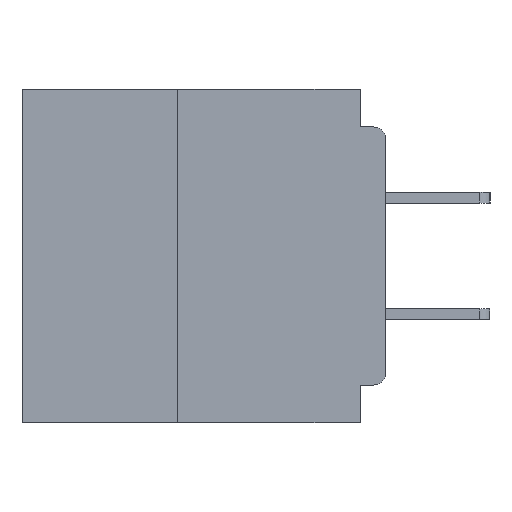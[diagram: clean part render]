
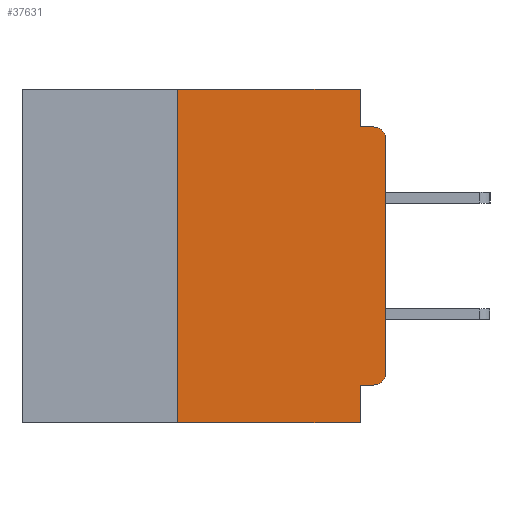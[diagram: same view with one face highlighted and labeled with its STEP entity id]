
A CAD part, left-side view. The second image highlights one B-rep face of the part: STEP entity #37631.
In plain terms, the highlighted planar face has unit normal (-1, 0, 0).
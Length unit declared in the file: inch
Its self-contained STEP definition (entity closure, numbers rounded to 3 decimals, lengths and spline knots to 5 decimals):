
#302 = DIRECTION ( 'NONE',  ( 0., 0., 1. ) ) ;
#959 = DIRECTION ( 'NONE',  ( 0., 0., -1. ) ) ;
#1338 = CARTESIAN_POINT ( 'NONE',  ( 0., 0.015, -0.045 ) ) ;
#1411 = ORIENTED_EDGE ( 'NONE', *, *, #16691, .T. ) ;
#1636 = VERTEX_POINT ( 'NONE', #13300 ) ;
#2552 = CARTESIAN_POINT ( 'NONE',  ( 0., 0.031, -0.4 ) ) ;
#2726 = VERTEX_POINT ( 'NONE', #1338 ) ;
#2742 = LINE ( 'NONE', #43406, #20763 ) ;
#3645 = VERTEX_POINT ( 'NONE', #13835 ) ;
#4211 = DIRECTION ( 'NONE',  ( 0., 0., -1. ) ) ;
#4636 = CARTESIAN_POINT ( 'NONE',  ( 0., 0.25, -0.4 ) ) ;
#4673 = CARTESIAN_POINT ( 'NONE',  ( 0., 0.031, 0. ) ) ;
#4762 = EDGE_CURVE ( 'NONE', #6671, #3645, #5255, .T. ) ;
#5042 = VECTOR ( 'NONE', #33403, 39.37008 ) ;
#5255 = LINE ( 'NONE', #2552, #23279 ) ;
#6236 = ORIENTED_EDGE ( 'NONE', *, *, #14813, .F. ) ;
#6671 = VERTEX_POINT ( 'NONE', #9232 ) ;
#7798 = ORIENTED_EDGE ( 'NONE', *, *, #25783, .T. ) ;
#8801 = DIRECTION ( 'NONE',  ( 0., 1., 0. ) ) ;
#9017 = VECTOR ( 'NONE', #30802, 39.37008 ) ;
#9232 = CARTESIAN_POINT ( 'NONE',  ( 0., 0.031, -0.355 ) ) ;
#9475 = AXIS2_PLACEMENT_3D ( 'NONE', #44064, #22482, #959 ) ;
#9657 = AXIS2_PLACEMENT_3D ( 'NONE', #11304, #25744, #4211 ) ;
#10311 = LINE ( 'NONE', #16710, #27148 ) ;
#11252 = LINE ( 'NONE', #22728, #5042 ) ;
#11304 = CARTESIAN_POINT ( 'NONE',  ( 0., 0.437, 0. ) ) ;
#11987 = LINE ( 'NONE', #4636, #20403 ) ;
#13208 = CARTESIAN_POINT ( 'NONE',  ( 0., 0.25, 0. ) ) ;
#13300 = CARTESIAN_POINT ( 'NONE',  ( 0., 0., -0.06 ) ) ;
#13835 = CARTESIAN_POINT ( 'NONE',  ( 0., 0.031, -0.4 ) ) ;
#14813 = EDGE_CURVE ( 'NONE', #42916, #33539, #35148, .T. ) ;
#16017 = VECTOR ( 'NONE', #8801, 39.37008 ) ;
#16586 = VERTEX_POINT ( 'NONE', #29084 ) ;
#16691 = EDGE_CURVE ( 'NONE', #1636, #2726, #40335, .T. ) ;
#16710 = CARTESIAN_POINT ( 'NONE',  ( 0., 0.437, 0. ) ) ;
#18535 = PLANE ( 'NONE',  #9657 ) ;
#18808 = VERTEX_POINT ( 'NONE', #13208 ) ;
#19559 = EDGE_CURVE ( 'NONE', #18808, #42916, #10311, .T. ) ;
#19618 = ORIENTED_EDGE ( 'NONE', *, *, #23415, .F. ) ;
#19667 = CARTESIAN_POINT ( 'NONE',  ( 0., 0.015, -0.355 ) ) ;
#20085 = CARTESIAN_POINT ( 'NONE',  ( 0., 0.015, -0.34 ) ) ;
#20403 = VECTOR ( 'NONE', #33405, 39.37008 ) ;
#20763 = VECTOR ( 'NONE', #302, 39.37008 ) ;
#20807 = EDGE_LOOP ( 'NONE', ( #30777, #1411, #39521, #6236, #39574, #31554, #7798, #27326, #19618, #28638 ) ) ;
#22482 = DIRECTION ( 'NONE',  ( -1., 0., 0. ) ) ;
#22728 = CARTESIAN_POINT ( 'NONE',  ( 0., 0., -0.045 ) ) ;
#23279 = VECTOR ( 'NONE', #24097, 39.37008 ) ;
#23415 = EDGE_CURVE ( 'NONE', #39044, #6671, #35107, .T. ) ;
#23688 = DIRECTION ( 'NONE',  ( 0., 0., -1. ) ) ;
#24097 = DIRECTION ( 'NONE',  ( 0., 0., -1. ) ) ;
#25744 = DIRECTION ( 'NONE',  ( 1., 0., 0. ) ) ;
#25758 = AXIS2_PLACEMENT_3D ( 'NONE', #20085, #45265, #23688 ) ;
#25783 = EDGE_CURVE ( 'NONE', #39995, #3645, #36567, .T. ) ;
#26922 = FACE_OUTER_BOUND ( 'NONE', #20807, .T. ) ;
#27148 = VECTOR ( 'NONE', #41887, 39.37008 ) ;
#27326 = ORIENTED_EDGE ( 'NONE', *, *, #4762, .F. ) ;
#28638 = ORIENTED_EDGE ( 'NONE', *, *, #42287, .T. ) ;
#29084 = CARTESIAN_POINT ( 'NONE',  ( 0., 0., -0.34 ) ) ;
#29939 = EDGE_CURVE ( 'NONE', #39995, #18808, #11987, .T. ) ;
#30314 = CARTESIAN_POINT ( 'NONE',  ( 0., 0., -0.355 ) ) ;
#30777 = ORIENTED_EDGE ( 'NONE', *, *, #37574, .T. ) ;
#30802 = DIRECTION ( 'NONE',  ( 0., -1., 0. ) ) ;
#31502 = EDGE_CURVE ( 'NONE', #33539, #2726, #11252, .T. ) ;
#31554 = ORIENTED_EDGE ( 'NONE', *, *, #29939, .F. ) ;
#31600 = CARTESIAN_POINT ( 'NONE',  ( 0., 0.25, -0.4 ) ) ;
#32938 = CIRCLE ( 'NONE', #25758, 0.015 ) ;
#33403 = DIRECTION ( 'NONE',  ( 0., -1., 0. ) ) ;
#33405 = DIRECTION ( 'NONE',  ( 0., 0., 1. ) ) ;
#33539 = VERTEX_POINT ( 'NONE', #34297 ) ;
#34006 = VECTOR ( 'NONE', #39203, 39.37008 ) ;
#34297 = CARTESIAN_POINT ( 'NONE',  ( 0., 0.031, -0.045 ) ) ;
#35107 = LINE ( 'NONE', #30314, #16017 ) ;
#35148 = LINE ( 'NONE', #42844, #34006 ) ;
#36567 = LINE ( 'NONE', #45136, #9017 ) ;
#37574 = EDGE_CURVE ( 'NONE', #16586, #1636, #2742, .T. ) ;
#37631 = ADVANCED_FACE ( 'NONE', ( #26922 ), #18535, .F. ) ;
#39044 = VERTEX_POINT ( 'NONE', #19667 ) ;
#39203 = DIRECTION ( 'NONE',  ( 0., 0., -1. ) ) ;
#39521 = ORIENTED_EDGE ( 'NONE', *, *, #31502, .F. ) ;
#39574 = ORIENTED_EDGE ( 'NONE', *, *, #19559, .F. ) ;
#39995 = VERTEX_POINT ( 'NONE', #31600 ) ;
#40335 = CIRCLE ( 'NONE', #9475, 0.015 ) ;
#41887 = DIRECTION ( 'NONE',  ( 0., -1., 0. ) ) ;
#42287 = EDGE_CURVE ( 'NONE', #39044, #16586, #32938, .T. ) ;
#42844 = CARTESIAN_POINT ( 'NONE',  ( 0., 0.031, 0. ) ) ;
#42916 = VERTEX_POINT ( 'NONE', #4673 ) ;
#43406 = CARTESIAN_POINT ( 'NONE',  ( 0., 0., 0. ) ) ;
#44064 = CARTESIAN_POINT ( 'NONE',  ( 0., 0.015, -0.06 ) ) ;
#45136 = CARTESIAN_POINT ( 'NONE',  ( 0., 0.437, -0.4 ) ) ;
#45265 = DIRECTION ( 'NONE',  ( -1., 0., 0. ) ) ;
